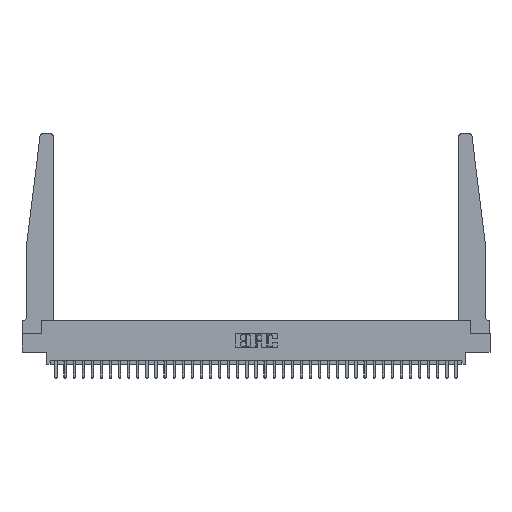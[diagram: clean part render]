
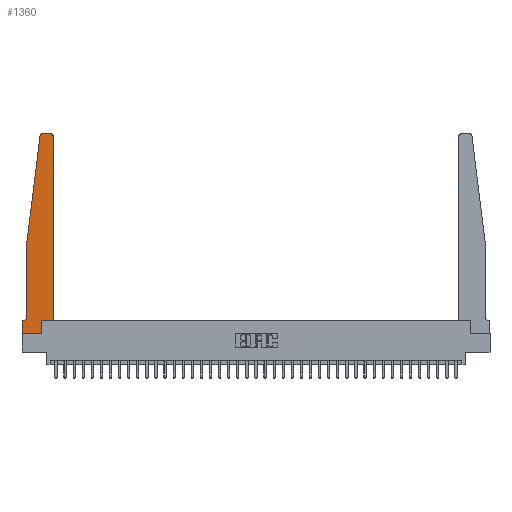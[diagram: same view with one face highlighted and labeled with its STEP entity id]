
A CAD part, top view. The second image highlights one B-rep face of the part: STEP entity #1360.
In plain terms, the highlighted planar face has unit normal (0, 0, 1).
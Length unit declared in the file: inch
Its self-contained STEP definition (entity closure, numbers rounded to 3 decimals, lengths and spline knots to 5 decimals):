
#146 = VERTEX_POINT ( 'NONE', #33993 ) ;
#215 = VECTOR ( 'NONE', #7541, 39.37008 ) ;
#895 = ORIENTED_EDGE ( 'NONE', *, *, #11634, .T. ) ;
#1095 = LINE ( 'NONE', #4763, #215 ) ;
#1274 = DIRECTION ( 'NONE',  ( -1., 0., 0. ) ) ;
#1360 = ADVANCED_FACE ( 'NONE', ( #11384 ), #20587, .T. ) ;
#1370 = VERTEX_POINT ( 'NONE', #30936 ) ;
#1391 = VERTEX_POINT ( 'NONE', #15384 ) ;
#1693 = CARTESIAN_POINT ( 'NONE',  ( 0.425, 0.18, 0.37 ) ) ;
#1734 = VERTEX_POINT ( 'NONE', #25318 ) ;
#2047 = VECTOR ( 'NONE', #27685, 39.37008 ) ;
#2556 = ORIENTED_EDGE ( 'NONE', *, *, #8749, .T. ) ;
#3499 = EDGE_CURVE ( 'NONE', #1734, #28819, #33181, .T. ) ;
#4107 = DIRECTION ( 'NONE',  ( 0., 0., 1. ) ) ;
#4662 = DIRECTION ( 'NONE',  ( 0., 0., 1. ) ) ;
#4763 = CARTESIAN_POINT ( 'NONE',  ( 0.25, 2.75, 0.37 ) ) ;
#5225 = VECTOR ( 'NONE', #20205, 39.37008 ) ;
#5524 = ORIENTED_EDGE ( 'NONE', *, *, #33310, .T. ) ;
#5691 = CARTESIAN_POINT ( 'NONE',  ( 0.425, 0.18, 0.37 ) ) ;
#6117 = LINE ( 'NONE', #17521, #5225 ) ;
#6279 = LINE ( 'NONE', #21995, #26426 ) ;
#6519 = EDGE_CURVE ( 'NONE', #17018, #25835, #20102, .T. ) ;
#7540 = VERTEX_POINT ( 'NONE', #13995 ) ;
#7541 = DIRECTION ( 'NONE',  ( -1., 0., 0. ) ) ;
#7791 = VERTEX_POINT ( 'NONE', #17789 ) ;
#8749 = EDGE_CURVE ( 'NONE', #25667, #146, #6279, .T. ) ;
#8914 = ORIENTED_EDGE ( 'NONE', *, *, #18692, .T. ) ;
#8985 = DIRECTION ( 'NONE',  ( -1., 0., 0. ) ) ;
#9809 = DIRECTION ( 'NONE',  ( 1., 0., 0. ) ) ;
#10750 = CARTESIAN_POINT ( 'NONE',  ( 0.27653, 2.75, 0.37 ) ) ;
#11384 = FACE_OUTER_BOUND ( 'NONE', #22739, .T. ) ;
#11634 = EDGE_CURVE ( 'NONE', #7540, #26408, #1095, .T. ) ;
#11791 = ORIENTED_EDGE ( 'NONE', *, *, #29319, .T. ) ;
#12109 = VECTOR ( 'NONE', #8985, 39.37008 ) ;
#12934 = EDGE_CURVE ( 'NONE', #28819, #1391, #6117, .T. ) ;
#13398 = ORIENTED_EDGE ( 'NONE', *, *, #12934, .T. ) ;
#13659 = CIRCLE ( 'NONE', #19001, 0.05 ) ;
#13838 = ORIENTED_EDGE ( 'NONE', *, *, #17325, .T. ) ;
#13995 = CARTESIAN_POINT ( 'NONE',  ( 0.395, 2.75, 0.37 ) ) ;
#14374 = CARTESIAN_POINT ( 'NONE',  ( 0.395, 2.72, 0.37 ) ) ;
#14434 = CARTESIAN_POINT ( 'NONE',  ( 0.2605, 0., 0.37 ) ) ;
#15384 = CARTESIAN_POINT ( 'NONE',  ( 0., 0., 0.37 ) ) ;
#16054 = CARTESIAN_POINT ( 'NONE',  ( 0.2605, 0.18, 0.37 ) ) ;
#16260 = LINE ( 'NONE', #24824, #29299 ) ;
#16721 = ORIENTED_EDGE ( 'NONE', *, *, #26090, .T. ) ;
#17018 = VERTEX_POINT ( 'NONE', #20990 ) ;
#17046 = DIRECTION ( 'NONE',  ( 1., 0., 0. ) ) ;
#17213 = LINE ( 'NONE', #25136, #23382 ) ;
#17237 = DIRECTION ( 'NONE',  ( 0., 0., -1. ) ) ;
#17325 = EDGE_CURVE ( 'NONE', #7791, #7540, #21019, .T. ) ;
#17521 = CARTESIAN_POINT ( 'NONE',  ( 0., 0., 0.37 ) ) ;
#17789 = CARTESIAN_POINT ( 'NONE',  ( 0.425, 2.72, 0.37 ) ) ;
#17793 = CARTESIAN_POINT ( 'NONE',  ( 0., 0.1875, 0.37 ) ) ;
#18331 = CARTESIAN_POINT ( 'NONE',  ( 0.24675, 2.72367, 0.37 ) ) ;
#18692 = EDGE_CURVE ( 'NONE', #146, #1370, #17213, .T. ) ;
#18733 = DIRECTION ( 'NONE',  ( 0., 1., 0. ) ) ;
#19001 = AXIS2_PLACEMENT_3D ( 'NONE', #32720, #17237, #1274 ) ;
#20054 = CARTESIAN_POINT ( 'NONE',  ( 0.27653, 2.72, 0.37 ) ) ;
#20102 = LINE ( 'NONE', #1693, #26174 ) ;
#20205 = DIRECTION ( 'NONE',  ( 0., -1., 0. ) ) ;
#20587 = PLANE ( 'NONE',  #32885 ) ;
#20990 = CARTESIAN_POINT ( 'NONE',  ( 0.2605, 0.18, 0.37 ) ) ;
#21019 = CIRCLE ( 'NONE', #32735, 0.03 ) ;
#21995 = CARTESIAN_POINT ( 'NONE',  ( 0.065, 1.25, 0.37 ) ) ;
#22095 = ORIENTED_EDGE ( 'NONE', *, *, #22626, .T. ) ;
#22517 = ORIENTED_EDGE ( 'NONE', *, *, #6519, .T. ) ;
#22626 = EDGE_CURVE ( 'NONE', #1370, #1734, #13659, .T. ) ;
#22659 = DIRECTION ( 'NONE',  ( 1., 0., 0. ) ) ;
#22739 = EDGE_LOOP ( 'NONE', ( #895, #16721, #2556, #8914, #22095, #27328, #13398, #5524, #11791, #22517, #27760, #13838 ) ) ;
#23200 = DIRECTION ( 'NONE',  ( 1., 0., 0. ) ) ;
#23209 = LINE ( 'NONE', #25104, #2047 ) ;
#23382 = VECTOR ( 'NONE', #27726, 39.37008 ) ;
#24824 = CARTESIAN_POINT ( 'NONE',  ( 0.425, 0.18, 0.37 ) ) ;
#25042 = CIRCLE ( 'NONE', #27112, 0.03 ) ;
#25104 = CARTESIAN_POINT ( 'NONE',  ( 0., 0., 0.37 ) ) ;
#25136 = CARTESIAN_POINT ( 'NONE',  ( 0.065, 1.25, 0.37 ) ) ;
#25318 = CARTESIAN_POINT ( 'NONE',  ( 0.015, 0.1875, 0.37 ) ) ;
#25667 = VERTEX_POINT ( 'NONE', #18331 ) ;
#25835 = VERTEX_POINT ( 'NONE', #5691 ) ;
#26090 = EDGE_CURVE ( 'NONE', #26408, #25667, #25042, .T. ) ;
#26174 = VECTOR ( 'NONE', #9809, 39.37008 ) ;
#26408 = VERTEX_POINT ( 'NONE', #10750 ) ;
#26426 = VECTOR ( 'NONE', #29651, 39.37008 ) ;
#27112 = AXIS2_PLACEMENT_3D ( 'NONE', #20054, #4107, #22659 ) ;
#27183 = CARTESIAN_POINT ( 'NONE',  ( 0.065, 0.1875, 0.37 ) ) ;
#27328 = ORIENTED_EDGE ( 'NONE', *, *, #3499, .T. ) ;
#27392 = DIRECTION ( 'NONE',  ( 0., 1., 0. ) ) ;
#27685 = DIRECTION ( 'NONE',  ( 1., 0., 0. ) ) ;
#27689 = LINE ( 'NONE', #16054, #33675 ) ;
#27726 = DIRECTION ( 'NONE',  ( 0., -1., 0. ) ) ;
#27760 = ORIENTED_EDGE ( 'NONE', *, *, #31619, .T. ) ;
#28819 = VERTEX_POINT ( 'NONE', #32056 ) ;
#29299 = VECTOR ( 'NONE', #27392, 39.37008 ) ;
#29319 = EDGE_CURVE ( 'NONE', #30402, #17018, #27689, .T. ) ;
#29651 = DIRECTION ( 'NONE',  ( -0.122, -0.992, 0. ) ) ;
#30402 = VERTEX_POINT ( 'NONE', #14434 ) ;
#30936 = CARTESIAN_POINT ( 'NONE',  ( 0.065, 0.2375, 0.37 ) ) ;
#31619 = EDGE_CURVE ( 'NONE', #25835, #7791, #16260, .T. ) ;
#32056 = CARTESIAN_POINT ( 'NONE',  ( 0., 0.1875, 0.37 ) ) ;
#32548 = DIRECTION ( 'NONE',  ( 0., 0., 1. ) ) ;
#32720 = CARTESIAN_POINT ( 'NONE',  ( 0.015, 0.2375, 0.37 ) ) ;
#32735 = AXIS2_PLACEMENT_3D ( 'NONE', #14374, #32548, #17046 ) ;
#32885 = AXIS2_PLACEMENT_3D ( 'NONE', #17793, #4662, #23200 ) ;
#33181 = LINE ( 'NONE', #27183, #12109 ) ;
#33310 = EDGE_CURVE ( 'NONE', #1391, #30402, #23209, .T. ) ;
#33675 = VECTOR ( 'NONE', #18733, 39.37008 ) ;
#33993 = CARTESIAN_POINT ( 'NONE',  ( 0.065, 1.25, 0.37 ) ) ;
